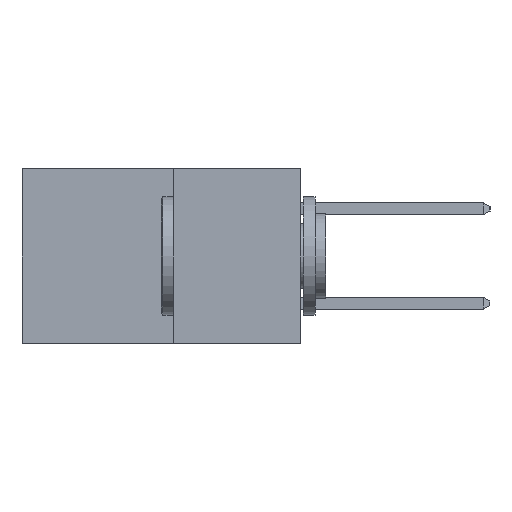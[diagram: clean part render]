
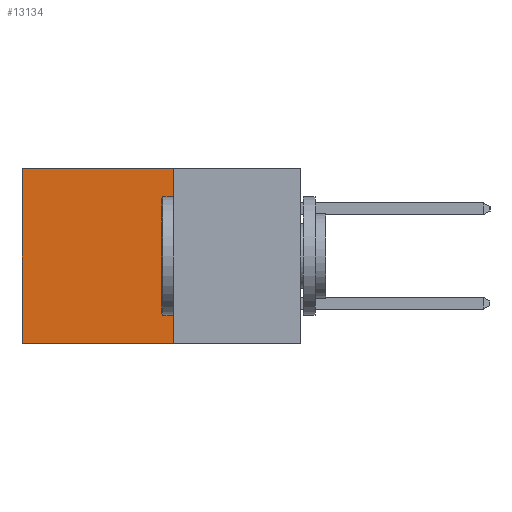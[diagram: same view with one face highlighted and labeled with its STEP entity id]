
A CAD part, left-side view. The second image highlights one B-rep face of the part: STEP entity #13134.
In plain terms, the highlighted planar face has unit normal (-1, 0, 0).
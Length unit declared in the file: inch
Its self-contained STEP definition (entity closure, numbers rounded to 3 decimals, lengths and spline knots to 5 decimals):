
#109 = CARTESIAN_POINT ( 'NONE',  ( 0.277, 0.59, -0.37 ) ) ;
#172 = ORIENTED_EDGE ( 'NONE', *, *, #13817, .F. ) ;
#1633 = DIRECTION ( 'NONE',  ( 0., 1., 0. ) ) ;
#1659 = DIRECTION ( 'NONE',  ( 0., 1., 0. ) ) ;
#2039 = EDGE_CURVE ( 'NONE', #9577, #15314, #15252, .T. ) ;
#3481 = DIRECTION ( 'NONE',  ( 0., 0., -1. ) ) ;
#4476 = DIRECTION ( 'NONE',  ( 0., 0., -1. ) ) ;
#4740 = CARTESIAN_POINT ( 'NONE',  ( 0.277, 0.59, -0.37 ) ) ;
#4886 = LINE ( 'NONE', #5208, #18450 ) ;
#5208 = CARTESIAN_POINT ( 'NONE',  ( 0.277, 0.27, -0.37 ) ) ;
#6064 = FACE_OUTER_BOUND ( 'NONE', #18324, .T. ) ;
#9132 = LINE ( 'NONE', #14226, #22549 ) ;
#9577 = VERTEX_POINT ( 'NONE', #19633 ) ;
#9737 = AXIS2_PLACEMENT_3D ( 'NONE', #19367, #14200, #3481 ) ;
#10122 = CARTESIAN_POINT ( 'NONE',  ( 0.277, 0.27, -0.37 ) ) ;
#10306 = LINE ( 'NONE', #12474, #19650 ) ;
#11655 = VERTEX_POINT ( 'NONE', #10122 ) ;
#11853 = ORIENTED_EDGE ( 'NONE', *, *, #2039, .T. ) ;
#12423 = PLANE ( 'NONE',  #9737 ) ;
#12474 = CARTESIAN_POINT ( 'NONE',  ( 0.277, 0.27, -0.37 ) ) ;
#13134 = ADVANCED_FACE ( 'NONE', ( #6064 ), #12423, .F. ) ;
#13817 = EDGE_CURVE ( 'NONE', #11655, #15314, #10306, .T. ) ;
#14200 = DIRECTION ( 'NONE',  ( 1., 0., 0. ) ) ;
#14226 = CARTESIAN_POINT ( 'NONE',  ( 0.277, 0.27, 0. ) ) ;
#14974 = VERTEX_POINT ( 'NONE', #16324 ) ;
#15252 = LINE ( 'NONE', #109, #19306 ) ;
#15314 = VERTEX_POINT ( 'NONE', #4740 ) ;
#16324 = CARTESIAN_POINT ( 'NONE',  ( 0.277, 0.27, 0. ) ) ;
#18240 = ORIENTED_EDGE ( 'NONE', *, *, #21214, .T. ) ;
#18324 = EDGE_LOOP ( 'NONE', ( #11853, #172, #21472, #18240 ) ) ;
#18450 = VECTOR ( 'NONE', #21014, 39.37008 ) ;
#19306 = VECTOR ( 'NONE', #4476, 39.37008 ) ;
#19367 = CARTESIAN_POINT ( 'NONE',  ( 0.277, 0.27, -0.37 ) ) ;
#19633 = CARTESIAN_POINT ( 'NONE',  ( 0.277, 0.59, 0. ) ) ;
#19650 = VECTOR ( 'NONE', #1659, 39.37008 ) ;
#21014 = DIRECTION ( 'NONE',  ( 0., 0., -1. ) ) ;
#21214 = EDGE_CURVE ( 'NONE', #14974, #9577, #9132, .T. ) ;
#21472 = ORIENTED_EDGE ( 'NONE', *, *, #22505, .F. ) ;
#22505 = EDGE_CURVE ( 'NONE', #14974, #11655, #4886, .T. ) ;
#22549 = VECTOR ( 'NONE', #1633, 39.37008 ) ;
